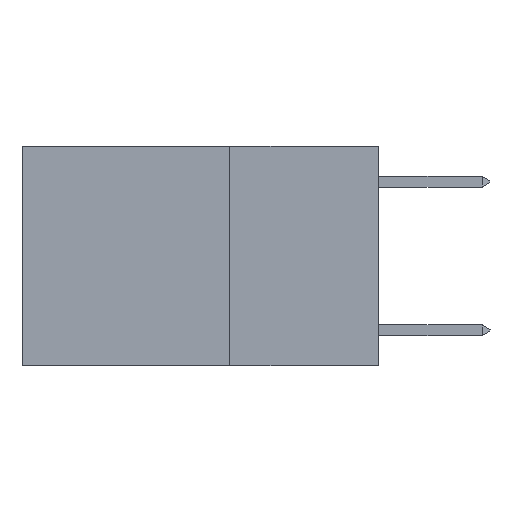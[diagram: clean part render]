
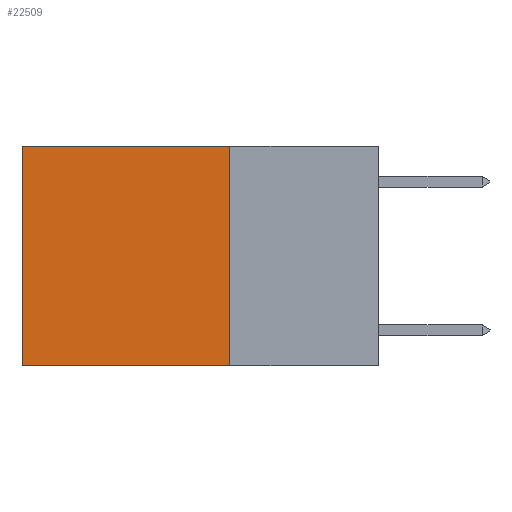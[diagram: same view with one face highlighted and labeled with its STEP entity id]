
A CAD part, left-side view. The second image highlights one B-rep face of the part: STEP entity #22509.
In plain terms, the highlighted planar face has unit normal (-1, 0, 0).
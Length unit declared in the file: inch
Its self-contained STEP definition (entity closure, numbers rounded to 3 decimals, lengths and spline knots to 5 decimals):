
#579 = CARTESIAN_POINT ( 'NONE',  ( 0.2625, 0.25, 0. ) ) ;
#716 = CARTESIAN_POINT ( 'NONE',  ( 0.2625, 0.25, -0.37 ) ) ;
#3587 = ORIENTED_EDGE ( 'NONE', *, *, #6545, .T. ) ;
#4869 = CARTESIAN_POINT ( 'NONE',  ( 0.2625, 0.6, 0. ) ) ;
#6197 = LINE ( 'NONE', #4869, #12344 ) ;
#6545 = EDGE_CURVE ( 'NONE', #12900, #7142, #14481, .T. ) ;
#6928 = VECTOR ( 'NONE', #25953, 39.37008 ) ;
#7088 = DIRECTION ( 'NONE',  ( 0., 0., -1. ) ) ;
#7142 = VERTEX_POINT ( 'NONE', #21373 ) ;
#7194 = PLANE ( 'NONE',  #11985 ) ;
#7813 = VECTOR ( 'NONE', #25927, 39.37008 ) ;
#9136 = CARTESIAN_POINT ( 'NONE',  ( 0.2625, 0.25, 0. ) ) ;
#9399 = CARTESIAN_POINT ( 'NONE',  ( 0.2625, 0.25, 0. ) ) ;
#10520 = EDGE_CURVE ( 'NONE', #7142, #21333, #6197, .T. ) ;
#11484 = ORIENTED_EDGE ( 'NONE', *, *, #12272, .F. ) ;
#11687 = EDGE_LOOP ( 'NONE', ( #21070, #18921, #11484, #3587 ) ) ;
#11851 = DIRECTION ( 'NONE',  ( 1., 0., 0. ) ) ;
#11985 = AXIS2_PLACEMENT_3D ( 'NONE', #9136, #11851, #7088 ) ;
#12272 = EDGE_CURVE ( 'NONE', #12900, #17686, #20077, .T. ) ;
#12344 = VECTOR ( 'NONE', #20488, 39.37008 ) ;
#12900 = VERTEX_POINT ( 'NONE', #9399 ) ;
#12988 = FACE_OUTER_BOUND ( 'NONE', #11687, .T. ) ;
#14481 = LINE ( 'NONE', #14542, #6928 ) ;
#14542 = CARTESIAN_POINT ( 'NONE',  ( 0.2625, 0.25, 0. ) ) ;
#14560 = CARTESIAN_POINT ( 'NONE',  ( 0.2625, 0.25, -0.37 ) ) ;
#17686 = VERTEX_POINT ( 'NONE', #14560 ) ;
#18921 = ORIENTED_EDGE ( 'NONE', *, *, #27570, .F. ) ;
#19123 = DIRECTION ( 'NONE',  ( 0., 0., -1. ) ) ;
#20077 = LINE ( 'NONE', #579, #26449 ) ;
#20488 = DIRECTION ( 'NONE',  ( 0., 0., -1. ) ) ;
#21070 = ORIENTED_EDGE ( 'NONE', *, *, #10520, .T. ) ;
#21242 = CARTESIAN_POINT ( 'NONE',  ( 0.2625, 0.6, -0.37 ) ) ;
#21333 = VERTEX_POINT ( 'NONE', #21242 ) ;
#21373 = CARTESIAN_POINT ( 'NONE',  ( 0.2625, 0.6, 0. ) ) ;
#22462 = LINE ( 'NONE', #716, #7813 ) ;
#22509 = ADVANCED_FACE ( 'NONE', ( #12988 ), #7194, .F. ) ;
#25927 = DIRECTION ( 'NONE',  ( 0., 1., 0. ) ) ;
#25953 = DIRECTION ( 'NONE',  ( 0., 1., 0. ) ) ;
#26449 = VECTOR ( 'NONE', #19123, 39.37008 ) ;
#27570 = EDGE_CURVE ( 'NONE', #17686, #21333, #22462, .T. ) ;
